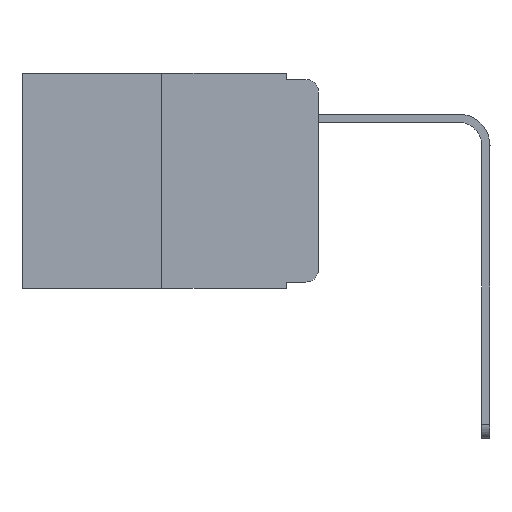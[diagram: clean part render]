
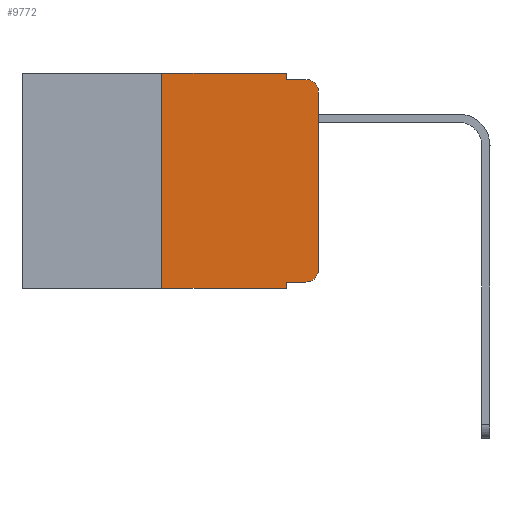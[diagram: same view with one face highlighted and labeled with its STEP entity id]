
A CAD part, left-side view. The second image highlights one B-rep face of the part: STEP entity #9772.
In plain terms, the highlighted planar face has unit normal (-1, 0, 0).
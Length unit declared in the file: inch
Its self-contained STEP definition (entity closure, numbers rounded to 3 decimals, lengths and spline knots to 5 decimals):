
#346 = CARTESIAN_POINT ( 'NONE',  ( 0., 0.051, -0.01 ) ) ;
#866 = DIRECTION ( 'NONE',  ( 0., 0., -1. ) ) ;
#1036 = VECTOR ( 'NONE', #10430, 39.37008 ) ;
#1213 = AXIS2_PLACEMENT_3D ( 'NONE', #21549, #23726, #866 ) ;
#1355 = CARTESIAN_POINT ( 'NONE',  ( 0., 0.25, -0.343 ) ) ;
#1917 = ORIENTED_EDGE ( 'NONE', *, *, #16982, .T. ) ;
#2481 = ORIENTED_EDGE ( 'NONE', *, *, #5796, .F. ) ;
#2604 = CARTESIAN_POINT ( 'NONE',  ( 0., 0.473, 0. ) ) ;
#3274 = DIRECTION ( 'NONE',  ( 0., 0., -1. ) ) ;
#3382 = DIRECTION ( 'NONE',  ( 0., -1., 0. ) ) ;
#4145 = CARTESIAN_POINT ( 'NONE',  ( 0., 0.051, -0.01 ) ) ;
#4374 = DIRECTION ( 'NONE',  ( 0., 0., 1. ) ) ;
#4574 = ORIENTED_EDGE ( 'NONE', *, *, #15232, .F. ) ;
#4657 = CIRCLE ( 'NONE', #11569, 0.02 ) ;
#5144 = AXIS2_PLACEMENT_3D ( 'NONE', #12212, #14124, #8713 ) ;
#5240 = DIRECTION ( 'NONE',  ( 0., -1., 0. ) ) ;
#5690 = ORIENTED_EDGE ( 'NONE', *, *, #23766, .T. ) ;
#5796 = EDGE_CURVE ( 'NONE', #8445, #15195, #12342, .T. ) ;
#5968 = CARTESIAN_POINT ( 'NONE',  ( 0., 0.25, 0. ) ) ;
#6053 = CARTESIAN_POINT ( 'NONE',  ( 0., 0., 0. ) ) ;
#7329 = CARTESIAN_POINT ( 'NONE',  ( 0., 0.051, -0.333 ) ) ;
#7473 = VECTOR ( 'NONE', #20866, 39.37008 ) ;
#7533 = CARTESIAN_POINT ( 'NONE',  ( 0., 0.051, 0. ) ) ;
#7542 = ORIENTED_EDGE ( 'NONE', *, *, #24072, .T. ) ;
#8044 = VECTOR ( 'NONE', #3382, 39.37008 ) ;
#8445 = VERTEX_POINT ( 'NONE', #1355 ) ;
#8479 = CARTESIAN_POINT ( 'NONE',  ( 0., 0.051, -0.333 ) ) ;
#8692 = FACE_OUTER_BOUND ( 'NONE', #21220, .T. ) ;
#8713 = DIRECTION ( 'NONE',  ( 0., 0., -1. ) ) ;
#8968 = CARTESIAN_POINT ( 'NONE',  ( 0., 0.02, -0.03 ) ) ;
#9743 = ORIENTED_EDGE ( 'NONE', *, *, #17560, .F. ) ;
#9772 = ADVANCED_FACE ( 'NONE', ( #8692 ), #13989, .F. ) ;
#10313 = CARTESIAN_POINT ( 'NONE',  ( 0., 0.051, 0. ) ) ;
#10430 = DIRECTION ( 'NONE',  ( 0., -1., 0. ) ) ;
#10889 = DIRECTION ( 'NONE',  ( -1., 0., 0. ) ) ;
#11069 = LINE ( 'NONE', #7533, #7473 ) ;
#11259 = CARTESIAN_POINT ( 'NONE',  ( 0., 0., -0.313 ) ) ;
#11292 = EDGE_CURVE ( 'NONE', #8445, #24584, #23953, .T. ) ;
#11322 = LINE ( 'NONE', #2604, #16074 ) ;
#11569 = AXIS2_PLACEMENT_3D ( 'NONE', #8968, #10889, #3274 ) ;
#11645 = EDGE_CURVE ( 'NONE', #15195, #24370, #11322, .T. ) ;
#11742 = VECTOR ( 'NONE', #24789, 39.37008 ) ;
#11832 = CARTESIAN_POINT ( 'NONE',  ( 0., 0., -0.03 ) ) ;
#12212 = CARTESIAN_POINT ( 'NONE',  ( 0., 0.02, -0.313 ) ) ;
#12342 = LINE ( 'NONE', #13524, #11742 ) ;
#12598 = VECTOR ( 'NONE', #4374, 39.37008 ) ;
#13268 = ORIENTED_EDGE ( 'NONE', *, *, #11292, .T. ) ;
#13524 = CARTESIAN_POINT ( 'NONE',  ( 0., 0.25, 0. ) ) ;
#13989 = PLANE ( 'NONE',  #1213 ) ;
#14124 = DIRECTION ( 'NONE',  ( -1., 0., 0. ) ) ;
#14164 = ORIENTED_EDGE ( 'NONE', *, *, #16705, .T. ) ;
#14828 = CARTESIAN_POINT ( 'NONE',  ( 0., 0.051, -0.343 ) ) ;
#14832 = CIRCLE ( 'NONE', #5144, 0.02 ) ;
#14835 = CARTESIAN_POINT ( 'NONE',  ( 0., 0.02, -0.333 ) ) ;
#14855 = CARTESIAN_POINT ( 'NONE',  ( 0., 0.02, -0.01 ) ) ;
#15195 = VERTEX_POINT ( 'NONE', #5968 ) ;
#15232 = EDGE_CURVE ( 'NONE', #16457, #24584, #17432, .T. ) ;
#15676 = DIRECTION ( 'NONE',  ( 0., 0., -1. ) ) ;
#15982 = DIRECTION ( 'NONE',  ( 0., -1., 0. ) ) ;
#16074 = VECTOR ( 'NONE', #15982, 39.37008 ) ;
#16457 = VERTEX_POINT ( 'NONE', #8479 ) ;
#16462 = ORIENTED_EDGE ( 'NONE', *, *, #11645, .F. ) ;
#16705 = EDGE_CURVE ( 'NONE', #22371, #17836, #4657, .T. ) ;
#16982 = EDGE_CURVE ( 'NONE', #22540, #17858, #14832, .T. ) ;
#17432 = LINE ( 'NONE', #21398, #20735 ) ;
#17560 = EDGE_CURVE ( 'NONE', #24823, #17836, #19289, .T. ) ;
#17836 = VERTEX_POINT ( 'NONE', #14855 ) ;
#17858 = VERTEX_POINT ( 'NONE', #11259 ) ;
#18319 = LINE ( 'NONE', #7329, #20998 ) ;
#18628 = CARTESIAN_POINT ( 'NONE',  ( 0., 0.473, -0.343 ) ) ;
#19289 = LINE ( 'NONE', #4145, #1036 ) ;
#19719 = ORIENTED_EDGE ( 'NONE', *, *, #24577, .F. ) ;
#20735 = VECTOR ( 'NONE', #15676, 39.37008 ) ;
#20866 = DIRECTION ( 'NONE',  ( 0., 0., -1. ) ) ;
#20998 = VECTOR ( 'NONE', #5240, 39.37008 ) ;
#21220 = EDGE_LOOP ( 'NONE', ( #7542, #14164, #9743, #19719, #16462, #2481, #13268, #4574, #5690, #1917 ) ) ;
#21398 = CARTESIAN_POINT ( 'NONE',  ( 0., 0.051, 0. ) ) ;
#21549 = CARTESIAN_POINT ( 'NONE',  ( 0., 0.473, 0. ) ) ;
#22371 = VERTEX_POINT ( 'NONE', #11832 ) ;
#22540 = VERTEX_POINT ( 'NONE', #14835 ) ;
#23404 = LINE ( 'NONE', #6053, #12598 ) ;
#23726 = DIRECTION ( 'NONE',  ( 1., 0., 0. ) ) ;
#23766 = EDGE_CURVE ( 'NONE', #16457, #22540, #18319, .T. ) ;
#23953 = LINE ( 'NONE', #18628, #8044 ) ;
#24072 = EDGE_CURVE ( 'NONE', #17858, #22371, #23404, .T. ) ;
#24370 = VERTEX_POINT ( 'NONE', #10313 ) ;
#24577 = EDGE_CURVE ( 'NONE', #24370, #24823, #11069, .T. ) ;
#24584 = VERTEX_POINT ( 'NONE', #14828 ) ;
#24789 = DIRECTION ( 'NONE',  ( 0., 0., 1. ) ) ;
#24823 = VERTEX_POINT ( 'NONE', #346 ) ;
